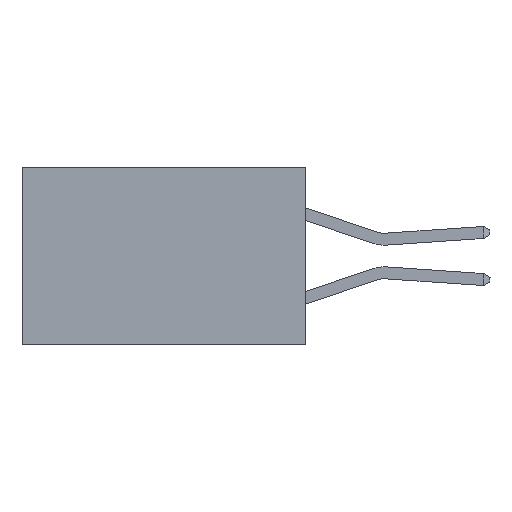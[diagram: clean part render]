
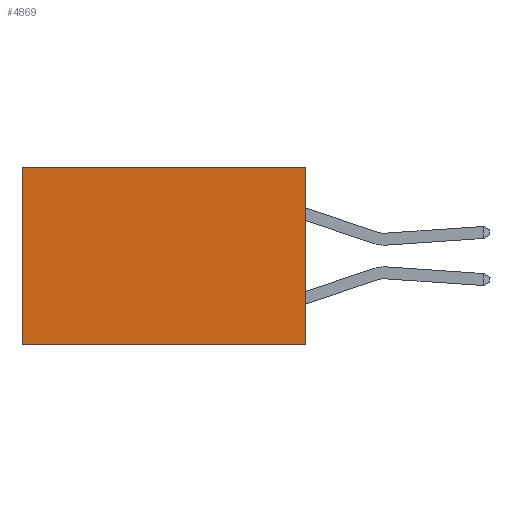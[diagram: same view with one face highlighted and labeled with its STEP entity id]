
A CAD part, left-side view. The second image highlights one B-rep face of the part: STEP entity #4869.
In plain terms, the highlighted planar face has unit normal (-1, 0, 0).
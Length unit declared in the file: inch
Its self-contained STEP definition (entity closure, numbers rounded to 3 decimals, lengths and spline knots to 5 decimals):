
#590 = VECTOR ( 'NONE', #10540, 39.37008 ) ;
#948 = DIRECTION ( 'NONE',  ( 0., 1., 0. ) ) ;
#2166 = CARTESIAN_POINT ( 'NONE',  ( 0.277, 0.59, 0. ) ) ;
#4869 = ADVANCED_FACE ( 'NONE', ( #22620 ), #18003, .F. ) ;
#6482 = CARTESIAN_POINT ( 'NONE',  ( 0.277, 0., 0. ) ) ;
#6936 = ORIENTED_EDGE ( 'NONE', *, *, #20963, .F. ) ;
#8034 = EDGE_LOOP ( 'NONE', ( #15730, #6936, #11938, #17499 ) ) ;
#9123 = DIRECTION ( 'NONE',  ( 0., 0., -1. ) ) ;
#9149 = CARTESIAN_POINT ( 'NONE',  ( 0.277, 0., -0.37 ) ) ;
#9288 = DIRECTION ( 'NONE',  ( 1., 0., 0. ) ) ;
#9655 = CARTESIAN_POINT ( 'NONE',  ( 0.277, 0., -0.37 ) ) ;
#9949 = VECTOR ( 'NONE', #23067, 39.37008 ) ;
#9993 = CARTESIAN_POINT ( 'NONE',  ( 0.277, 0.59, -0.37 ) ) ;
#10381 = EDGE_CURVE ( 'NONE', #12531, #17533, #14639, .T. ) ;
#10536 = LINE ( 'NONE', #19868, #590 ) ;
#10540 = DIRECTION ( 'NONE',  ( 0., 1., 0. ) ) ;
#11070 = DIRECTION ( 'NONE',  ( 0., 0., -1. ) ) ;
#11938 = ORIENTED_EDGE ( 'NONE', *, *, #18644, .F. ) ;
#12006 = VERTEX_POINT ( 'NONE', #19941 ) ;
#12531 = VERTEX_POINT ( 'NONE', #6482 ) ;
#12940 = VERTEX_POINT ( 'NONE', #22413 ) ;
#12992 = VECTOR ( 'NONE', #11070, 39.37008 ) ;
#14639 = LINE ( 'NONE', #17816, #19054 ) ;
#15730 = ORIENTED_EDGE ( 'NONE', *, *, #23495, .T. ) ;
#17400 = LINE ( 'NONE', #9149, #12992 ) ;
#17499 = ORIENTED_EDGE ( 'NONE', *, *, #10381, .T. ) ;
#17533 = VERTEX_POINT ( 'NONE', #2166 ) ;
#17816 = CARTESIAN_POINT ( 'NONE',  ( 0.277, 0., 0. ) ) ;
#18003 = PLANE ( 'NONE',  #18769 ) ;
#18644 = EDGE_CURVE ( 'NONE', #12531, #12006, #17400, .T. ) ;
#18769 = AXIS2_PLACEMENT_3D ( 'NONE', #9655, #9288, #9123 ) ;
#19054 = VECTOR ( 'NONE', #948, 39.37008 ) ;
#19337 = LINE ( 'NONE', #9993, #9949 ) ;
#19868 = CARTESIAN_POINT ( 'NONE',  ( 0.277, 0., -0.37 ) ) ;
#19941 = CARTESIAN_POINT ( 'NONE',  ( 0.277, 0., -0.37 ) ) ;
#20963 = EDGE_CURVE ( 'NONE', #12006, #12940, #10536, .T. ) ;
#22413 = CARTESIAN_POINT ( 'NONE',  ( 0.277, 0.59, -0.37 ) ) ;
#22620 = FACE_OUTER_BOUND ( 'NONE', #8034, .T. ) ;
#23067 = DIRECTION ( 'NONE',  ( 0., 0., -1. ) ) ;
#23495 = EDGE_CURVE ( 'NONE', #17533, #12940, #19337, .T. ) ;
